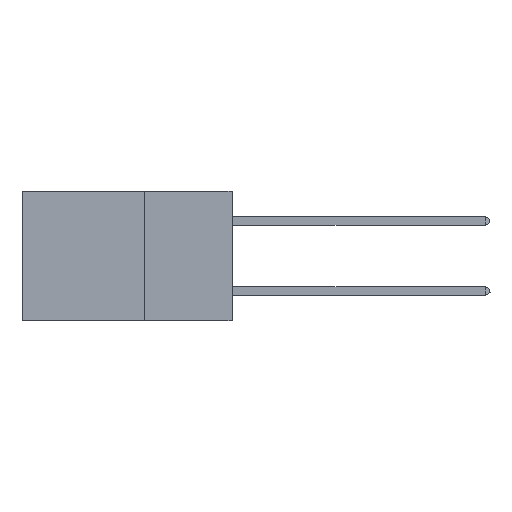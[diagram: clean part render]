
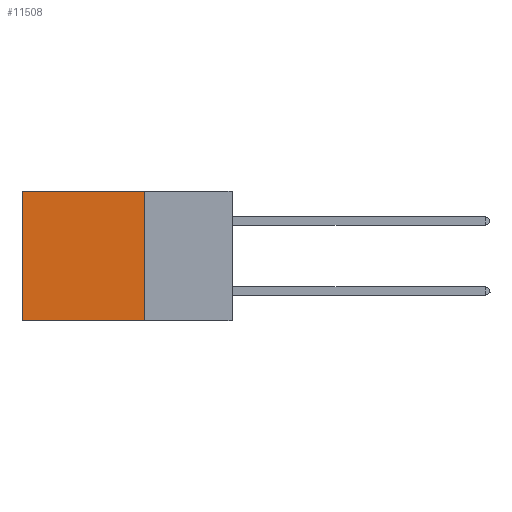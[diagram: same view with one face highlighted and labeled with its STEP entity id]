
A CAD part, left-side view. The second image highlights one B-rep face of the part: STEP entity #11508.
In plain terms, the highlighted planar face has unit normal (-1, 0, 0).
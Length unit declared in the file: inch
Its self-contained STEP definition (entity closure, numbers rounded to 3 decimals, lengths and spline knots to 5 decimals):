
#132 = VERTEX_POINT ( 'NONE', #21916 ) ;
#149 = DIRECTION ( 'NONE',  ( 0., 0., -1. ) ) ;
#245 = CARTESIAN_POINT ( 'NONE',  ( 0.2875, 0.25, 0. ) ) ;
#1202 = ORIENTED_EDGE ( 'NONE', *, *, #29302, .F. ) ;
#3383 = AXIS2_PLACEMENT_3D ( 'NONE', #7789, #12769, #21931 ) ;
#3925 = CARTESIAN_POINT ( 'NONE',  ( 0.2875, 0.6, 0. ) ) ;
#5977 = VERTEX_POINT ( 'NONE', #23676 ) ;
#7271 = VERTEX_POINT ( 'NONE', #16292 ) ;
#7388 = ORIENTED_EDGE ( 'NONE', *, *, #11923, .F. ) ;
#7738 = CARTESIAN_POINT ( 'NONE',  ( 0.2875, 0.25, -0.37 ) ) ;
#7789 = CARTESIAN_POINT ( 'NONE',  ( 0.2875, 0.25, 0. ) ) ;
#7879 = DIRECTION ( 'NONE',  ( 0., 1., 0. ) ) ;
#7904 = CARTESIAN_POINT ( 'NONE',  ( 0.2875, 0.6, 0. ) ) ;
#9214 = LINE ( 'NONE', #7738, #20496 ) ;
#10255 = DIRECTION ( 'NONE',  ( 0., 0., -1. ) ) ;
#11508 = ADVANCED_FACE ( 'NONE', ( #24306 ), #17195, .F. ) ;
#11923 = EDGE_CURVE ( 'NONE', #5977, #7271, #17765, .T. ) ;
#12453 = CARTESIAN_POINT ( 'NONE',  ( 0.2875, 0.25, 0. ) ) ;
#12769 = DIRECTION ( 'NONE',  ( 1., 0., 0. ) ) ;
#12844 = ORIENTED_EDGE ( 'NONE', *, *, #26588, .T. ) ;
#13563 = VECTOR ( 'NONE', #10255, 39.37008 ) ;
#14098 = LINE ( 'NONE', #12453, #22428 ) ;
#15172 = VECTOR ( 'NONE', #149, 39.37008 ) ;
#16292 = CARTESIAN_POINT ( 'NONE',  ( 0.2875, 0.25, -0.37 ) ) ;
#17043 = DIRECTION ( 'NONE',  ( 0., 1., 0. ) ) ;
#17195 = PLANE ( 'NONE',  #3383 ) ;
#17765 = LINE ( 'NONE', #245, #15172 ) ;
#20043 = ORIENTED_EDGE ( 'NONE', *, *, #23449, .T. ) ;
#20420 = VERTEX_POINT ( 'NONE', #3925 ) ;
#20496 = VECTOR ( 'NONE', #17043, 39.37008 ) ;
#21916 = CARTESIAN_POINT ( 'NONE',  ( 0.2875, 0.6, -0.37 ) ) ;
#21931 = DIRECTION ( 'NONE',  ( 0., 0., -1. ) ) ;
#22428 = VECTOR ( 'NONE', #7879, 39.37008 ) ;
#22570 = EDGE_LOOP ( 'NONE', ( #12844, #1202, #7388, #20043 ) ) ;
#23449 = EDGE_CURVE ( 'NONE', #5977, #20420, #14098, .T. ) ;
#23676 = CARTESIAN_POINT ( 'NONE',  ( 0.2875, 0.25, 0. ) ) ;
#24306 = FACE_OUTER_BOUND ( 'NONE', #22570, .T. ) ;
#25947 = LINE ( 'NONE', #7904, #13563 ) ;
#26588 = EDGE_CURVE ( 'NONE', #20420, #132, #25947, .T. ) ;
#29302 = EDGE_CURVE ( 'NONE', #7271, #132, #9214, .T. ) ;
